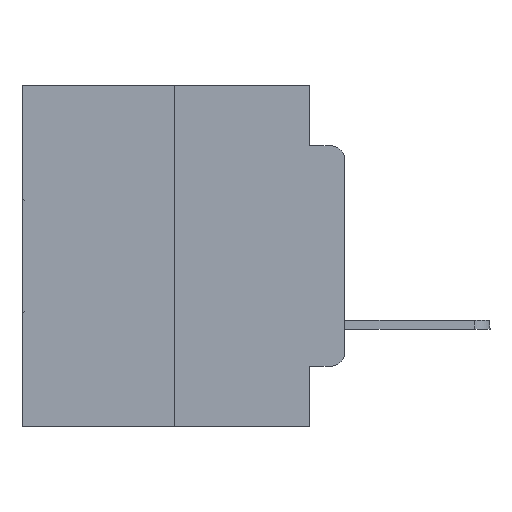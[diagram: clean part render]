
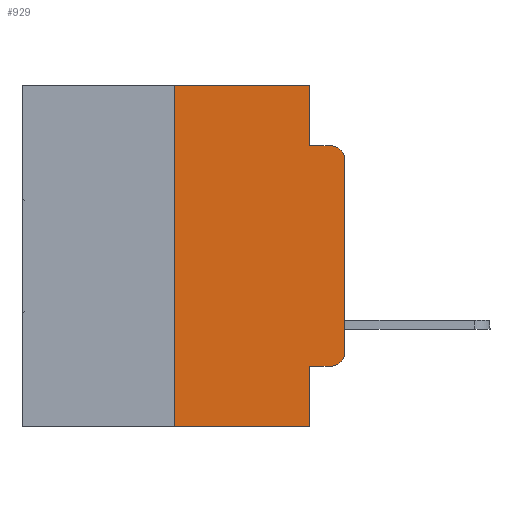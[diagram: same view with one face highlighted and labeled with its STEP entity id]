
A CAD part, left-side view. The second image highlights one B-rep face of the part: STEP entity #929.
In plain terms, the highlighted planar face has unit normal (-1, 0, 0).
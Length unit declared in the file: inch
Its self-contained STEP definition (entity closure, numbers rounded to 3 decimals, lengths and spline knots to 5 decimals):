
#396 = DIRECTION ( 'NONE',  ( 0., 0., -1. ) ) ;
#893 = DIRECTION ( 'NONE',  ( 0., 0., 1. ) ) ;
#898 = VECTOR ( 'NONE', #893, 39.37008 ) ;
#929 = ADVANCED_FACE ( 'NONE', ( #16418 ), #18672, .F. ) ;
#1315 = CARTESIAN_POINT ( 'NONE',  ( 0., 0.02, -0.3915 ) ) ;
#1959 = LINE ( 'NONE', #6358, #23651 ) ;
#1984 = CARTESIAN_POINT ( 'NONE',  ( 0., 0., -0.1085 ) ) ;
#2012 = ORIENTED_EDGE ( 'NONE', *, *, #2743, .F. ) ;
#2477 = CARTESIAN_POINT ( 'NONE',  ( 0., 0.25, 0. ) ) ;
#2507 = VERTEX_POINT ( 'NONE', #19509 ) ;
#2606 = CARTESIAN_POINT ( 'NONE',  ( 0., 0.051, -0.0885 ) ) ;
#2743 = EDGE_CURVE ( 'NONE', #8739, #6092, #13470, .T. ) ;
#2797 = DIRECTION ( 'NONE',  ( 0., 0., -1. ) ) ;
#3099 = DIRECTION ( 'NONE',  ( 1., 0., 0. ) ) ;
#3192 = ORIENTED_EDGE ( 'NONE', *, *, #18838, .F. ) ;
#3286 = CIRCLE ( 'NONE', #11503, 0.02 ) ;
#4251 = CARTESIAN_POINT ( 'NONE',  ( 0., 0.25, 0. ) ) ;
#4688 = CARTESIAN_POINT ( 'NONE',  ( 0., 0.051, 0. ) ) ;
#4692 = VERTEX_POINT ( 'NONE', #6874 ) ;
#5175 = CARTESIAN_POINT ( 'NONE',  ( 0., 0.473, -0.5 ) ) ;
#5313 = EDGE_CURVE ( 'NONE', #8739, #8412, #25843, .T. ) ;
#5699 = ORIENTED_EDGE ( 'NONE', *, *, #27859, .T. ) ;
#5909 = AXIS2_PLACEMENT_3D ( 'NONE', #21071, #3099, #10059 ) ;
#6092 = VERTEX_POINT ( 'NONE', #2477 ) ;
#6146 = CARTESIAN_POINT ( 'NONE',  ( 0., 0.473, 0. ) ) ;
#6255 = ORIENTED_EDGE ( 'NONE', *, *, #29797, .F. ) ;
#6358 = CARTESIAN_POINT ( 'NONE',  ( 0., 0., 0. ) ) ;
#6419 = VECTOR ( 'NONE', #28935, 39.37008 ) ;
#6671 = LINE ( 'NONE', #4688, #23399 ) ;
#6874 = CARTESIAN_POINT ( 'NONE',  ( 0., 0., -0.3915 ) ) ;
#7068 = CARTESIAN_POINT ( 'NONE',  ( 0., 0.25, -0.5 ) ) ;
#7560 = EDGE_CURVE ( 'NONE', #23586, #4692, #13024, .T. ) ;
#7694 = VECTOR ( 'NONE', #14369, 39.37008 ) ;
#7944 = DIRECTION ( 'NONE',  ( -1., 0., 0. ) ) ;
#8412 = VERTEX_POINT ( 'NONE', #19592 ) ;
#8514 = EDGE_CURVE ( 'NONE', #22739, #23586, #18229, .T. ) ;
#8739 = VERTEX_POINT ( 'NONE', #7068 ) ;
#8753 = DIRECTION ( 'NONE',  ( 0., 0., 1. ) ) ;
#9450 = CARTESIAN_POINT ( 'NONE',  ( 0., 0.051, 0. ) ) ;
#10059 = DIRECTION ( 'NONE',  ( 0., 0., -1. ) ) ;
#10181 = EDGE_CURVE ( 'NONE', #6092, #24734, #28786, .T. ) ;
#10513 = DIRECTION ( 'NONE',  ( 0., 0., -1. ) ) ;
#11503 = AXIS2_PLACEMENT_3D ( 'NONE', #13821, #20762, #2797 ) ;
#11734 = CARTESIAN_POINT ( 'NONE',  ( 0., 0.02, -0.4115 ) ) ;
#12014 = LINE ( 'NONE', #9450, #23385 ) ;
#12463 = VERTEX_POINT ( 'NONE', #1984 ) ;
#13024 = CIRCLE ( 'NONE', #26508, 0.02 ) ;
#13470 = LINE ( 'NONE', #4251, #898 ) ;
#13821 = CARTESIAN_POINT ( 'NONE',  ( 0., 0.02, -0.1085 ) ) ;
#14369 = DIRECTION ( 'NONE',  ( 0., -1., 0. ) ) ;
#14513 = VECTOR ( 'NONE', #25086, 39.37008 ) ;
#15130 = CARTESIAN_POINT ( 'NONE',  ( 0., 0.051, 0. ) ) ;
#15887 = CARTESIAN_POINT ( 'NONE',  ( 0., 0.051, -0.0885 ) ) ;
#16178 = ORIENTED_EDGE ( 'NONE', *, *, #24053, .T. ) ;
#16322 = ORIENTED_EDGE ( 'NONE', *, *, #8514, .T. ) ;
#16418 = FACE_OUTER_BOUND ( 'NONE', #22386, .T. ) ;
#16444 = VECTOR ( 'NONE', #29555, 39.37008 ) ;
#16813 = ORIENTED_EDGE ( 'NONE', *, *, #27444, .F. ) ;
#18229 = LINE ( 'NONE', #29407, #16444 ) ;
#18672 = PLANE ( 'NONE',  #5909 ) ;
#18838 = EDGE_CURVE ( 'NONE', #24734, #24434, #12014, .T. ) ;
#19509 = CARTESIAN_POINT ( 'NONE',  ( 0., 0.02, -0.0885 ) ) ;
#19592 = CARTESIAN_POINT ( 'NONE',  ( 0., 0.051, -0.5 ) ) ;
#20762 = DIRECTION ( 'NONE',  ( -1., 0., 0. ) ) ;
#20917 = ORIENTED_EDGE ( 'NONE', *, *, #7560, .T. ) ;
#21071 = CARTESIAN_POINT ( 'NONE',  ( 0., 0.473, 0. ) ) ;
#22386 = EDGE_LOOP ( 'NONE', ( #5699, #16178, #16813, #3192, #28825, #2012, #24357, #6255, #16322, #20917 ) ) ;
#22739 = VERTEX_POINT ( 'NONE', #23317 ) ;
#22960 = DIRECTION ( 'NONE',  ( 0., 0., -1. ) ) ;
#23317 = CARTESIAN_POINT ( 'NONE',  ( 0., 0.051, -0.4115 ) ) ;
#23385 = VECTOR ( 'NONE', #396, 39.37008 ) ;
#23399 = VECTOR ( 'NONE', #22960, 39.37008 ) ;
#23586 = VERTEX_POINT ( 'NONE', #11734 ) ;
#23651 = VECTOR ( 'NONE', #8753, 39.37008 ) ;
#24053 = EDGE_CURVE ( 'NONE', #12463, #2507, #3286, .T. ) ;
#24357 = ORIENTED_EDGE ( 'NONE', *, *, #5313, .T. ) ;
#24434 = VERTEX_POINT ( 'NONE', #2606 ) ;
#24734 = VERTEX_POINT ( 'NONE', #15130 ) ;
#25086 = DIRECTION ( 'NONE',  ( 0., -1., 0. ) ) ;
#25843 = LINE ( 'NONE', #5175, #7694 ) ;
#26508 = AXIS2_PLACEMENT_3D ( 'NONE', #1315, #7944, #10513 ) ;
#27054 = LINE ( 'NONE', #15887, #14513 ) ;
#27444 = EDGE_CURVE ( 'NONE', #24434, #2507, #27054, .T. ) ;
#27859 = EDGE_CURVE ( 'NONE', #4692, #12463, #1959, .T. ) ;
#28786 = LINE ( 'NONE', #6146, #6419 ) ;
#28825 = ORIENTED_EDGE ( 'NONE', *, *, #10181, .F. ) ;
#28935 = DIRECTION ( 'NONE',  ( 0., -1., 0. ) ) ;
#29407 = CARTESIAN_POINT ( 'NONE',  ( 0., 0.051, -0.4115 ) ) ;
#29555 = DIRECTION ( 'NONE',  ( 0., -1., 0. ) ) ;
#29797 = EDGE_CURVE ( 'NONE', #22739, #8412, #6671, .T. ) ;
